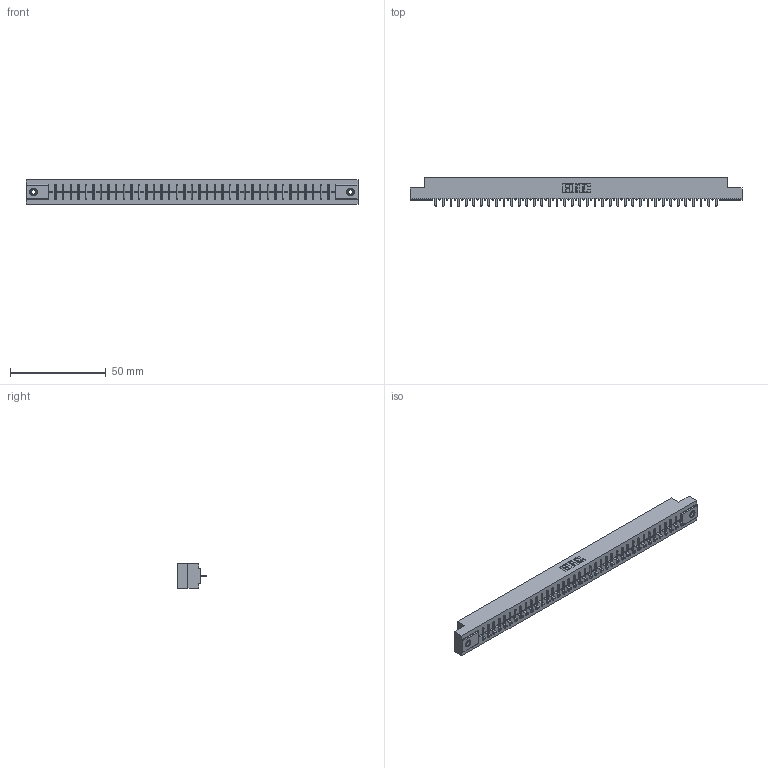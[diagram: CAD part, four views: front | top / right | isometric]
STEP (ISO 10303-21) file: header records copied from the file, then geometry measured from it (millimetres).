
FILE_DESCRIPTION (( 'STEP AP203' ), '1' );
FILE_NAME ('306-038-521-108.STEP', '2019-09-12T00:02:25', ( '' ), ( '' ), 'SwSTEP 2.0', 'SolidWorks 2016', '' );
FILE_SCHEMA (( 'CONFIG_CONTROL_DESIGN' ));
Length unit declared in the file: inch
Products named in the file (4): 306 Part_.156 Dia; 306-038-521-108; 306-290-001_121; 345-250-001_345-250-003-102
Assembly tree (41 placements, depth 2):
  306-038-521-108
    306 Part_.156 Dia
    306-290-001_121  x38
    345-250-001_345-250-003-102  x2
Bounding box: 173.58 x 14.88 x 12.7 mm (x, y, z)
Volume: 19103.7 mm3; surface area: 19314.5 mm2
Topology: 41 solids, 41 shells, 2836 faces, 7938 edges, 5080 vertices
Faces by surface type: plane 1886, cylinder 782, sphere 152, cone 12, torus 4
Entity records: 37096 total; most frequent: CARTESIAN_POINT 6208, ORIENTED_EDGE 6148, DIRECTION 6130, EDGE_CURVE 3074, LINE 2402, VECTOR 2402, VERTEX_POINT 1942, AXIS2_PLACEMENT_3D 1864
